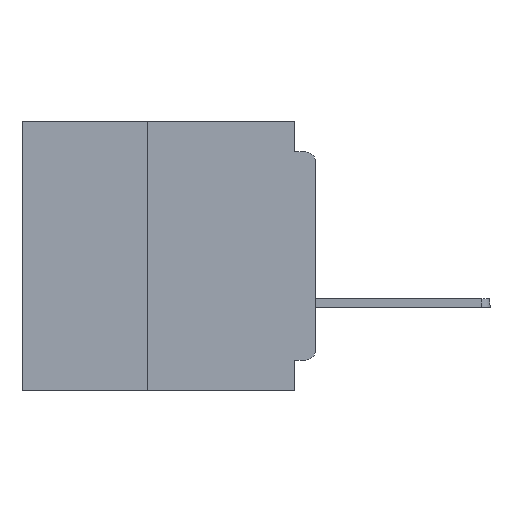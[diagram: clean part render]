
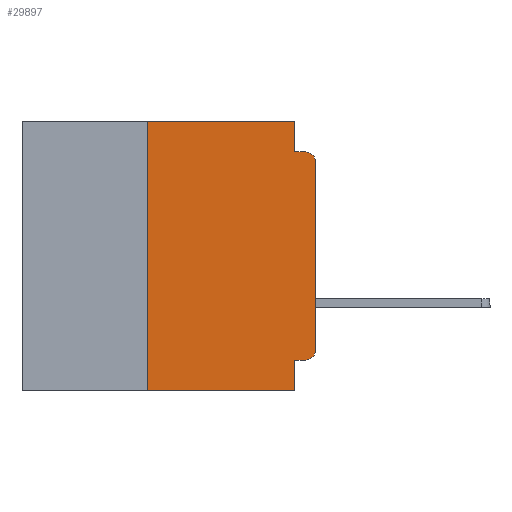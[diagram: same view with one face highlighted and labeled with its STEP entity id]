
A CAD part, left-side view. The second image highlights one B-rep face of the part: STEP entity #29897.
In plain terms, the highlighted planar face has unit normal (-1, 0, 0).
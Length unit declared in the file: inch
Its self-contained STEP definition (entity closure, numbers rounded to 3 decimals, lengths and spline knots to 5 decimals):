
#653 = CARTESIAN_POINT ( 'NONE',  ( 0., 0.25, -0.4 ) ) ;
#816 = CARTESIAN_POINT ( 'NONE',  ( 0., 0.015, -0.045 ) ) ;
#3002 = CIRCLE ( 'NONE', #21220, 0.015 ) ;
#3673 = CARTESIAN_POINT ( 'NONE',  ( 0., 0., -0.06 ) ) ;
#3695 = EDGE_CURVE ( 'NONE', #13324, #51056, #11995, .T. ) ;
#3941 = CARTESIAN_POINT ( 'NONE',  ( 0., 0.437, -0.4 ) ) ;
#4079 = VERTEX_POINT ( 'NONE', #31742 ) ;
#4114 = ORIENTED_EDGE ( 'NONE', *, *, #41793, .T. ) ;
#4332 = PLANE ( 'NONE',  #24169 ) ;
#5541 = CARTESIAN_POINT ( 'NONE',  ( 0., 0.015, -0.06 ) ) ;
#5840 = CARTESIAN_POINT ( 'NONE',  ( 0., 0.031, -0.045 ) ) ;
#6644 = VERTEX_POINT ( 'NONE', #5840 ) ;
#8317 = CARTESIAN_POINT ( 'NONE',  ( 0., 0.437, 0. ) ) ;
#8726 = ORIENTED_EDGE ( 'NONE', *, *, #10992, .F. ) ;
#8796 = DIRECTION ( 'NONE',  ( 0., 0., -1. ) ) ;
#9857 = DIRECTION ( 'NONE',  ( -1., 0., 0. ) ) ;
#10004 = DIRECTION ( 'NONE',  ( 0., 0., -1. ) ) ;
#10992 = EDGE_CURVE ( 'NONE', #20906, #4079, #56416, .T. ) ;
#11115 = ORIENTED_EDGE ( 'NONE', *, *, #41938, .F. ) ;
#11595 = CARTESIAN_POINT ( 'NONE',  ( 0., 0., -0.045 ) ) ;
#11777 = DIRECTION ( 'NONE',  ( 0., 0., 1. ) ) ;
#11995 = LINE ( 'NONE', #14768, #55583 ) ;
#12942 = VECTOR ( 'NONE', #26133, 39.37008 ) ;
#13324 = VERTEX_POINT ( 'NONE', #25799 ) ;
#13521 = VERTEX_POINT ( 'NONE', #816 ) ;
#14383 = DIRECTION ( 'NONE',  ( 0., 1., 0. ) ) ;
#14768 = CARTESIAN_POINT ( 'NONE',  ( 0., 0., -0.355 ) ) ;
#15001 = ORIENTED_EDGE ( 'NONE', *, *, #48662, .F. ) ;
#16043 = DIRECTION ( 'NONE',  ( 0., -1., 0. ) ) ;
#16220 = CARTESIAN_POINT ( 'NONE',  ( 0., 0., 0. ) ) ;
#16673 = EDGE_LOOP ( 'NONE', ( #31741, #4114, #11115, #15001, #8726, #19914, #54197, #47084, #22413, #21391 ) ) ;
#17184 = CARTESIAN_POINT ( 'NONE',  ( 0., 0.25, -0.4 ) ) ;
#17244 = DIRECTION ( 'NONE',  ( 0., -1., 0. ) ) ;
#17281 = EDGE_CURVE ( 'NONE', #21578, #25975, #44593, .T. ) ;
#18009 = VECTOR ( 'NONE', #29471, 39.37008 ) ;
#19391 = VECTOR ( 'NONE', #50621, 39.37008 ) ;
#19914 = ORIENTED_EDGE ( 'NONE', *, *, #26634, .F. ) ;
#20369 = LINE ( 'NONE', #17184, #53583 ) ;
#20467 = VECTOR ( 'NONE', #17244, 39.37008 ) ;
#20906 = VERTEX_POINT ( 'NONE', #42927 ) ;
#21175 = EDGE_CURVE ( 'NONE', #13324, #21578, #47636, .T. ) ;
#21220 = AXIS2_PLACEMENT_3D ( 'NONE', #5541, #36207, #10004 ) ;
#21391 = ORIENTED_EDGE ( 'NONE', *, *, #21175, .T. ) ;
#21578 = VERTEX_POINT ( 'NONE', #56329 ) ;
#22413 = ORIENTED_EDGE ( 'NONE', *, *, #3695, .F. ) ;
#24169 = AXIS2_PLACEMENT_3D ( 'NONE', #39221, #34996, #8796 ) ;
#25129 = CARTESIAN_POINT ( 'NONE',  ( 0., 0.031, -0.4 ) ) ;
#25799 = CARTESIAN_POINT ( 'NONE',  ( 0., 0.015, -0.355 ) ) ;
#25975 = VERTEX_POINT ( 'NONE', #3673 ) ;
#26133 = DIRECTION ( 'NONE',  ( 0., -1., 0. ) ) ;
#26634 = EDGE_CURVE ( 'NONE', #52315, #20906, #20369, .T. ) ;
#27143 = VECTOR ( 'NONE', #16043, 39.37008 ) ;
#28151 = EDGE_CURVE ( 'NONE', #52315, #48428, #47744, .T. ) ;
#28500 = LINE ( 'NONE', #11595, #27143 ) ;
#29471 = DIRECTION ( 'NONE',  ( 0., 0., -1. ) ) ;
#29677 = AXIS2_PLACEMENT_3D ( 'NONE', #36061, #9857, #40437 ) ;
#29897 = ADVANCED_FACE ( 'NONE', ( #54944 ), #4332, .F. ) ;
#31741 = ORIENTED_EDGE ( 'NONE', *, *, #17281, .T. ) ;
#31742 = CARTESIAN_POINT ( 'NONE',  ( 0., 0.031, 0. ) ) ;
#34996 = DIRECTION ( 'NONE',  ( 1., 0., 0. ) ) ;
#36061 = CARTESIAN_POINT ( 'NONE',  ( 0., 0.015, -0.34 ) ) ;
#36207 = DIRECTION ( 'NONE',  ( -1., 0., 0. ) ) ;
#39221 = CARTESIAN_POINT ( 'NONE',  ( 0., 0.437, 0. ) ) ;
#40437 = DIRECTION ( 'NONE',  ( 0., 0., -1. ) ) ;
#41793 = EDGE_CURVE ( 'NONE', #25975, #13521, #3002, .T. ) ;
#41938 = EDGE_CURVE ( 'NONE', #6644, #13521, #28500, .T. ) ;
#42927 = CARTESIAN_POINT ( 'NONE',  ( 0., 0.25, 0. ) ) ;
#43226 = VECTOR ( 'NONE', #11777, 39.37008 ) ;
#43237 = DIRECTION ( 'NONE',  ( 0., 0., 1. ) ) ;
#44593 = LINE ( 'NONE', #16220, #43226 ) ;
#46256 = CARTESIAN_POINT ( 'NONE',  ( 0., 0.031, 0. ) ) ;
#47084 = ORIENTED_EDGE ( 'NONE', *, *, #49384, .F. ) ;
#47636 = CIRCLE ( 'NONE', #29677, 0.015 ) ;
#47744 = LINE ( 'NONE', #3941, #12942 ) ;
#48428 = VERTEX_POINT ( 'NONE', #53270 ) ;
#48662 = EDGE_CURVE ( 'NONE', #4079, #6644, #53975, .T. ) ;
#49384 = EDGE_CURVE ( 'NONE', #51056, #48428, #51295, .T. ) ;
#50621 = DIRECTION ( 'NONE',  ( 0., 0., -1. ) ) ;
#51056 = VERTEX_POINT ( 'NONE', #52864 ) ;
#51295 = LINE ( 'NONE', #25129, #18009 ) ;
#52315 = VERTEX_POINT ( 'NONE', #653 ) ;
#52864 = CARTESIAN_POINT ( 'NONE',  ( 0., 0.031, -0.355 ) ) ;
#53270 = CARTESIAN_POINT ( 'NONE',  ( 0., 0.031, -0.4 ) ) ;
#53583 = VECTOR ( 'NONE', #43237, 39.37008 ) ;
#53975 = LINE ( 'NONE', #46256, #19391 ) ;
#54197 = ORIENTED_EDGE ( 'NONE', *, *, #28151, .T. ) ;
#54944 = FACE_OUTER_BOUND ( 'NONE', #16673, .T. ) ;
#55583 = VECTOR ( 'NONE', #14383, 39.37008 ) ;
#56329 = CARTESIAN_POINT ( 'NONE',  ( 0., 0., -0.34 ) ) ;
#56416 = LINE ( 'NONE', #8317, #20467 ) ;
